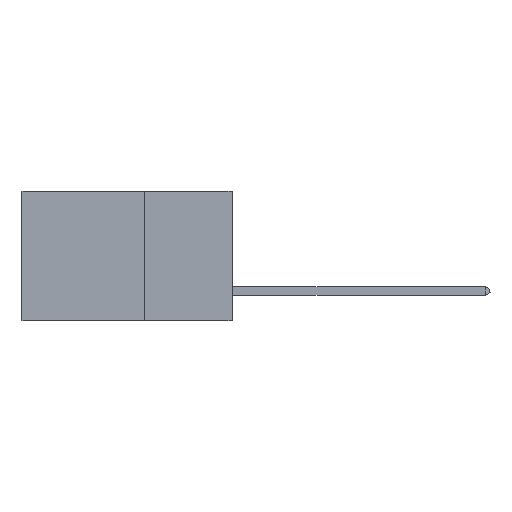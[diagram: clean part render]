
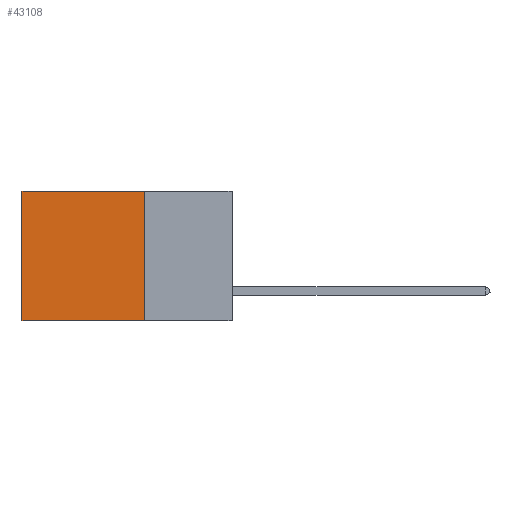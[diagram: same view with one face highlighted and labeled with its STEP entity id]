
A CAD part, left-side view. The second image highlights one B-rep face of the part: STEP entity #43108.
In plain terms, the highlighted planar face has unit normal (-1, 0, 0).
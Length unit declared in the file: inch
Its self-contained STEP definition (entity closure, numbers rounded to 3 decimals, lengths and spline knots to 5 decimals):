
#750 = DIRECTION ( 'NONE',  ( 0., 1., 0. ) ) ;
#1558 = DIRECTION ( 'NONE',  ( 0., 1., 0. ) ) ;
#2724 = DIRECTION ( 'NONE',  ( 0., 0., -1. ) ) ;
#2966 = EDGE_CURVE ( 'NONE', #18383, #35631, #16776, .T. ) ;
#3459 = VERTEX_POINT ( 'NONE', #40762 ) ;
#4414 = CARTESIAN_POINT ( 'NONE',  ( 0.2875, 0.25, 0. ) ) ;
#5415 = VECTOR ( 'NONE', #1558, 39.37008 ) ;
#6258 = CARTESIAN_POINT ( 'NONE',  ( 0.2875, 0.6, 0. ) ) ;
#6388 = DIRECTION ( 'NONE',  ( 1., 0., 0. ) ) ;
#7665 = CARTESIAN_POINT ( 'NONE',  ( 0.2875, 0.6, 0. ) ) ;
#7801 = EDGE_CURVE ( 'NONE', #19640, #35631, #41495, .T. ) ;
#9693 = LINE ( 'NONE', #4414, #37795 ) ;
#10262 = DIRECTION ( 'NONE',  ( 0., 0., -1. ) ) ;
#16776 = LINE ( 'NONE', #20888, #5415 ) ;
#16922 = ORIENTED_EDGE ( 'NONE', *, *, #7801, .T. ) ;
#17423 = CARTESIAN_POINT ( 'NONE',  ( 0.2875, 0.6, -0.37 ) ) ;
#18383 = VERTEX_POINT ( 'NONE', #48017 ) ;
#19178 = DIRECTION ( 'NONE',  ( 0., 0., -1. ) ) ;
#19640 = VERTEX_POINT ( 'NONE', #6258 ) ;
#20888 = CARTESIAN_POINT ( 'NONE',  ( 0.2875, 0.25, -0.37 ) ) ;
#22047 = CARTESIAN_POINT ( 'NONE',  ( 0.2875, 0.25, 0. ) ) ;
#26466 = EDGE_CURVE ( 'NONE', #3459, #18383, #29832, .T. ) ;
#28657 = VECTOR ( 'NONE', #2724, 39.37008 ) ;
#28800 = VECTOR ( 'NONE', #19178, 39.37008 ) ;
#29832 = LINE ( 'NONE', #22047, #28657 ) ;
#31746 = FACE_OUTER_BOUND ( 'NONE', #33471, .T. ) ;
#33471 = EDGE_LOOP ( 'NONE', ( #16922, #34657, #42596, #47900 ) ) ;
#34657 = ORIENTED_EDGE ( 'NONE', *, *, #2966, .F. ) ;
#35201 = AXIS2_PLACEMENT_3D ( 'NONE', #48773, #6388, #10262 ) ;
#35631 = VERTEX_POINT ( 'NONE', #17423 ) ;
#37477 = PLANE ( 'NONE',  #35201 ) ;
#37795 = VECTOR ( 'NONE', #750, 39.37008 ) ;
#40762 = CARTESIAN_POINT ( 'NONE',  ( 0.2875, 0.25, 0. ) ) ;
#41495 = LINE ( 'NONE', #7665, #28800 ) ;
#42596 = ORIENTED_EDGE ( 'NONE', *, *, #26466, .F. ) ;
#43108 = ADVANCED_FACE ( 'NONE', ( #31746 ), #37477, .F. ) ;
#47900 = ORIENTED_EDGE ( 'NONE', *, *, #48329, .T. ) ;
#48017 = CARTESIAN_POINT ( 'NONE',  ( 0.2875, 0.25, -0.37 ) ) ;
#48329 = EDGE_CURVE ( 'NONE', #3459, #19640, #9693, .T. ) ;
#48773 = CARTESIAN_POINT ( 'NONE',  ( 0.2875, 0.25, 0. ) ) ;
